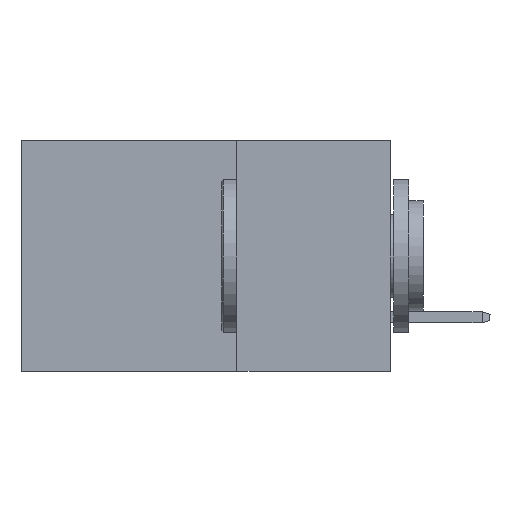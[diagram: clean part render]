
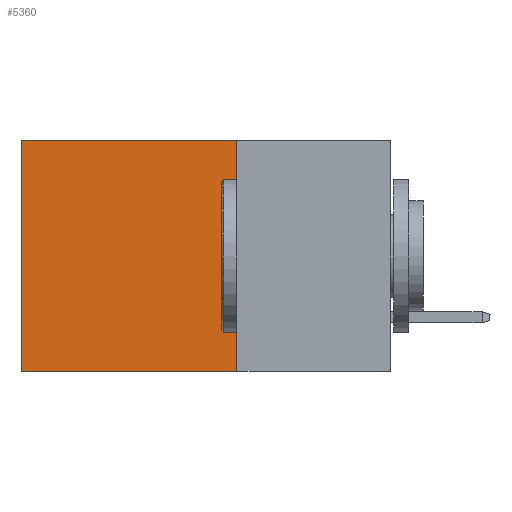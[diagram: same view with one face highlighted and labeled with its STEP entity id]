
A CAD part, left-side view. The second image highlights one B-rep face of the part: STEP entity #5360.
In plain terms, the highlighted planar face has unit normal (-1, 0, 0).
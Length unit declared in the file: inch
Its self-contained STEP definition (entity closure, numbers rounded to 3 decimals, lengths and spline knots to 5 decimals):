
#230 = PLANE ( 'NONE',  #6224 ) ;
#318 = VERTEX_POINT ( 'NONE', #4950 ) ;
#536 = EDGE_CURVE ( 'NONE', #7783, #2929, #7556, .T. ) ;
#746 = CARTESIAN_POINT ( 'NONE',  ( 0.2875, 0.25, -0.375 ) ) ;
#1169 = VECTOR ( 'NONE', #3009, 39.37008 ) ;
#1288 = DIRECTION ( 'NONE',  ( 0., 1., 0. ) ) ;
#1775 = ORIENTED_EDGE ( 'NONE', *, *, #536, .F. ) ;
#1777 = EDGE_CURVE ( 'NONE', #318, #2929, #7756, .T. ) ;
#1948 = VECTOR ( 'NONE', #4494, 39.37008 ) ;
#2027 = VECTOR ( 'NONE', #1288, 39.37008 ) ;
#2183 = CARTESIAN_POINT ( 'NONE',  ( 0.2875, 0.6, -0.375 ) ) ;
#2929 = VERTEX_POINT ( 'NONE', #5928 ) ;
#2964 = VERTEX_POINT ( 'NONE', #7420 ) ;
#3009 = DIRECTION ( 'NONE',  ( 0., 0., -1. ) ) ;
#3109 = EDGE_CURVE ( 'NONE', #2964, #318, #6740, .T. ) ;
#3146 = CARTESIAN_POINT ( 'NONE',  ( 0.2875, 0.25, -0.375 ) ) ;
#3293 = ORIENTED_EDGE ( 'NONE', *, *, #1777, .T. ) ;
#3697 = CARTESIAN_POINT ( 'NONE',  ( 0.2875, 0.25, -0.375 ) ) ;
#3835 = FACE_OUTER_BOUND ( 'NONE', #5028, .T. ) ;
#4358 = ORIENTED_EDGE ( 'NONE', *, *, #6831, .F. ) ;
#4452 = LINE ( 'NONE', #5866, #1169 ) ;
#4494 = DIRECTION ( 'NONE',  ( 0., 1., 0. ) ) ;
#4804 = CARTESIAN_POINT ( 'NONE',  ( 0.2875, 0.25, 0. ) ) ;
#4950 = CARTESIAN_POINT ( 'NONE',  ( 0.2875, 0.6, 0. ) ) ;
#5028 = EDGE_LOOP ( 'NONE', ( #3293, #1775, #4358, #5636 ) ) ;
#5360 = ADVANCED_FACE ( 'NONE', ( #3835 ), #230, .F. ) ;
#5636 = ORIENTED_EDGE ( 'NONE', *, *, #3109, .T. ) ;
#5866 = CARTESIAN_POINT ( 'NONE',  ( 0.2875, 0.25, -0.375 ) ) ;
#5928 = CARTESIAN_POINT ( 'NONE',  ( 0.2875, 0.6, -0.375 ) ) ;
#6224 = AXIS2_PLACEMENT_3D ( 'NONE', #3697, #6505, #7459 ) ;
#6505 = DIRECTION ( 'NONE',  ( 1., 0., 0. ) ) ;
#6740 = LINE ( 'NONE', #4804, #2027 ) ;
#6831 = EDGE_CURVE ( 'NONE', #2964, #7783, #4452, .T. ) ;
#7420 = CARTESIAN_POINT ( 'NONE',  ( 0.2875, 0.25, 0. ) ) ;
#7459 = DIRECTION ( 'NONE',  ( 0., 0., -1. ) ) ;
#7556 = LINE ( 'NONE', #3146, #1948 ) ;
#7756 = LINE ( 'NONE', #2183, #8833 ) ;
#7783 = VERTEX_POINT ( 'NONE', #746 ) ;
#8418 = DIRECTION ( 'NONE',  ( 0., 0., -1. ) ) ;
#8833 = VECTOR ( 'NONE', #8418, 39.37008 ) ;
